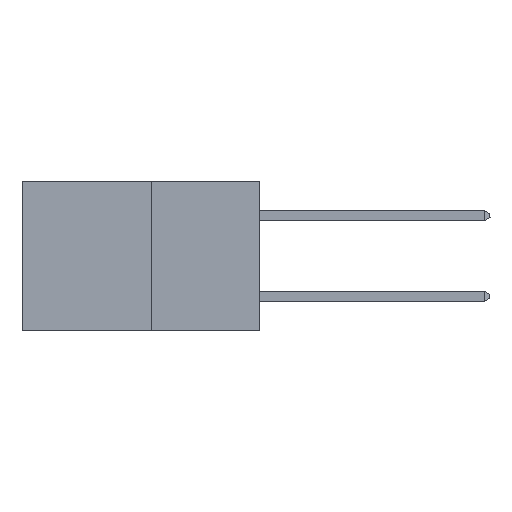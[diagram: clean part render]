
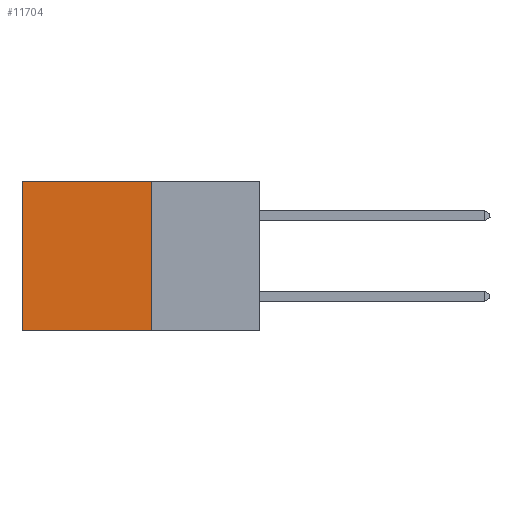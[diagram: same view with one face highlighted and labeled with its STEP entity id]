
A CAD part, left-side view. The second image highlights one B-rep face of the part: STEP entity #11704.
In plain terms, the highlighted planar face has unit normal (-1, 0, 0).
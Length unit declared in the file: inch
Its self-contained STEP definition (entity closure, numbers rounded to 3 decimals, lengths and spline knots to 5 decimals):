
#181 = CARTESIAN_POINT ( 'NONE',  ( 0.277, 0.27, -0.37 ) ) ;
#1619 = EDGE_CURVE ( 'NONE', #8698, #12257, #14514, .T. ) ;
#1663 = EDGE_CURVE ( 'NONE', #14966, #11393, #13132, .T. ) ;
#2030 = LINE ( 'NONE', #8124, #5169 ) ;
#2276 = CARTESIAN_POINT ( 'NONE',  ( 0.277, 0.59, -0.37 ) ) ;
#2922 = CARTESIAN_POINT ( 'NONE',  ( 0.277, 0.59, 0. ) ) ;
#3188 = DIRECTION ( 'NONE',  ( 0., 1., 0. ) ) ;
#4268 = ORIENTED_EDGE ( 'NONE', *, *, #1663, .F. ) ;
#4514 = EDGE_CURVE ( 'NONE', #14966, #8698, #2030, .T. ) ;
#4609 = VECTOR ( 'NONE', #3188, 39.37008 ) ;
#4779 = CARTESIAN_POINT ( 'NONE',  ( 0.277, 0.27, -0.37 ) ) ;
#5169 = VECTOR ( 'NONE', #8214, 39.37008 ) ;
#5502 = ORIENTED_EDGE ( 'NONE', *, *, #1619, .T. ) ;
#5857 = ORIENTED_EDGE ( 'NONE', *, *, #9683, .F. ) ;
#5897 = PLANE ( 'NONE',  #12415 ) ;
#7068 = DIRECTION ( 'NONE',  ( 1., 0., 0. ) ) ;
#7319 = ORIENTED_EDGE ( 'NONE', *, *, #4514, .T. ) ;
#8124 = CARTESIAN_POINT ( 'NONE',  ( 0.277, 0.27, 0. ) ) ;
#8214 = DIRECTION ( 'NONE',  ( 0., 1., 0. ) ) ;
#8698 = VERTEX_POINT ( 'NONE', #2922 ) ;
#8948 = CARTESIAN_POINT ( 'NONE',  ( 0.277, 0.27, -0.37 ) ) ;
#9048 = DIRECTION ( 'NONE',  ( 0., 0., -1. ) ) ;
#9683 = EDGE_CURVE ( 'NONE', #11393, #12257, #10758, .T. ) ;
#9945 = FACE_OUTER_BOUND ( 'NONE', #12235, .T. ) ;
#10095 = VECTOR ( 'NONE', #9048, 39.37008 ) ;
#10758 = LINE ( 'NONE', #8948, #4609 ) ;
#11393 = VERTEX_POINT ( 'NONE', #11785 ) ;
#11459 = CARTESIAN_POINT ( 'NONE',  ( 0.277, 0.59, -0.37 ) ) ;
#11704 = ADVANCED_FACE ( 'NONE', ( #9945 ), #5897, .F. ) ;
#11785 = CARTESIAN_POINT ( 'NONE',  ( 0.277, 0.27, -0.37 ) ) ;
#12235 = EDGE_LOOP ( 'NONE', ( #5502, #5857, #4268, #7319 ) ) ;
#12257 = VERTEX_POINT ( 'NONE', #11459 ) ;
#12415 = AXIS2_PLACEMENT_3D ( 'NONE', #4779, #7068, #15030 ) ;
#13132 = LINE ( 'NONE', #181, #10095 ) ;
#14166 = VECTOR ( 'NONE', #15031, 39.37008 ) ;
#14385 = CARTESIAN_POINT ( 'NONE',  ( 0.277, 0.27, 0. ) ) ;
#14514 = LINE ( 'NONE', #2276, #14166 ) ;
#14966 = VERTEX_POINT ( 'NONE', #14385 ) ;
#15030 = DIRECTION ( 'NONE',  ( 0., 0., -1. ) ) ;
#15031 = DIRECTION ( 'NONE',  ( 0., 0., -1. ) ) ;
